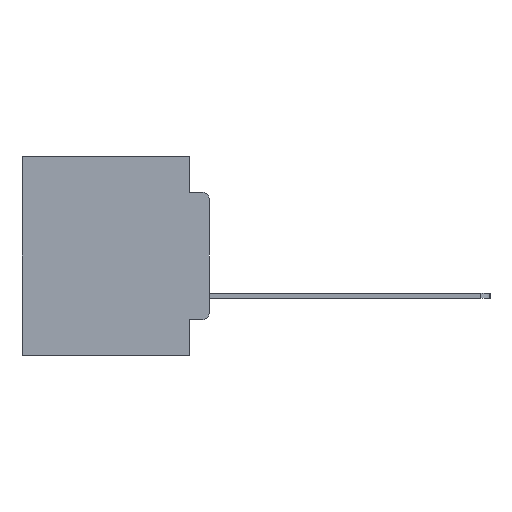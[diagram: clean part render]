
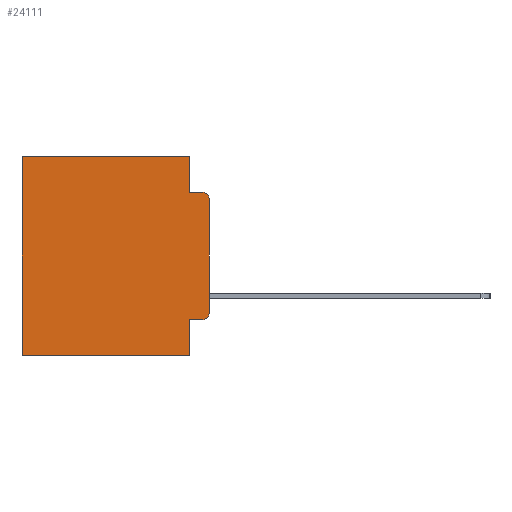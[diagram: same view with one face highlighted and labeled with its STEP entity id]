
A CAD part, left-side view. The second image highlights one B-rep face of the part: STEP entity #24111.
In plain terms, the highlighted planar face has unit normal (-1, 0, 0).
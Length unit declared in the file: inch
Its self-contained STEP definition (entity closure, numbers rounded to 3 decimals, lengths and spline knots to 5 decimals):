
#613 = CIRCLE ( 'NONE', #1823, 0.02 ) ;
#683 = ORIENTED_EDGE ( 'NONE', *, *, #22437, .F. ) ;
#1132 = CARTESIAN_POINT ( 'NONE',  ( 0.298, 0.473, -0.5 ) ) ;
#1179 = LINE ( 'NONE', #14755, #17703 ) ;
#1577 = AXIS2_PLACEMENT_3D ( 'NONE', #6906, #22453, #9178 ) ;
#1823 = AXIS2_PLACEMENT_3D ( 'NONE', #12701, #28021, #14940 ) ;
#1908 = LINE ( 'NONE', #10897, #24934 ) ;
#2142 = ORIENTED_EDGE ( 'NONE', *, *, #2997, .T. ) ;
#2168 = VERTEX_POINT ( 'NONE', #1132 ) ;
#2997 = EDGE_CURVE ( 'NONE', #19765, #2168, #7782, .T. ) ;
#3572 = ORIENTED_EDGE ( 'NONE', *, *, #9066, .F. ) ;
#4216 = DIRECTION ( 'NONE',  ( 0., 1., 0. ) ) ;
#4220 = EDGE_CURVE ( 'NONE', #27204, #19765, #25929, .T. ) ;
#4390 = DIRECTION ( 'NONE',  ( 0., 0., -1. ) ) ;
#4971 = CARTESIAN_POINT ( 'NONE',  ( 0.298, 0., 0. ) ) ;
#5161 = VECTOR ( 'NONE', #7639, 39.37008 ) ;
#5734 = AXIS2_PLACEMENT_3D ( 'NONE', #4971, #20560, #7235 ) ;
#6906 = CARTESIAN_POINT ( 'NONE',  ( 0.298, 0.02, -0.3915 ) ) ;
#7235 = DIRECTION ( 'NONE',  ( 0., 0., -1. ) ) ;
#7298 = CARTESIAN_POINT ( 'NONE',  ( 0.298, 0.051, -0.5 ) ) ;
#7639 = DIRECTION ( 'NONE',  ( 0., 0., -1. ) ) ;
#7782 = LINE ( 'NONE', #15590, #18922 ) ;
#8420 = CARTESIAN_POINT ( 'NONE',  ( 0.298, 0.473, 0. ) ) ;
#8427 = CARTESIAN_POINT ( 'NONE',  ( 0.298, 0.051, -0.0885 ) ) ;
#8883 = EDGE_CURVE ( 'NONE', #19855, #25365, #18760, .T. ) ;
#8916 = VECTOR ( 'NONE', #24172, 39.37008 ) ;
#9066 = EDGE_CURVE ( 'NONE', #27204, #15815, #1908, .T. ) ;
#9178 = DIRECTION ( 'NONE',  ( 0., 0., -1. ) ) ;
#9445 = CARTESIAN_POINT ( 'NONE',  ( 0.298, 0.02, -0.0885 ) ) ;
#9495 = CIRCLE ( 'NONE', #1577, 0.02 ) ;
#10897 = CARTESIAN_POINT ( 'NONE',  ( 0.298, 0.051, 0. ) ) ;
#11019 = ORIENTED_EDGE ( 'NONE', *, *, #20965, .T. ) ;
#11169 = LINE ( 'NONE', #23171, #5161 ) ;
#11352 = ORIENTED_EDGE ( 'NONE', *, *, #26916, .T. ) ;
#12701 = CARTESIAN_POINT ( 'NONE',  ( 0.298, 0.02, -0.1085 ) ) ;
#12762 = ORIENTED_EDGE ( 'NONE', *, *, #19210, .F. ) ;
#14160 = CARTESIAN_POINT ( 'NONE',  ( 0.298, 0., -0.3915 ) ) ;
#14560 = CARTESIAN_POINT ( 'NONE',  ( 0.298, 0.051, 0. ) ) ;
#14755 = CARTESIAN_POINT ( 'NONE',  ( 0.298, 0.051, -0.0885 ) ) ;
#14853 = ORIENTED_EDGE ( 'NONE', *, *, #4220, .T. ) ;
#14940 = DIRECTION ( 'NONE',  ( 0., 0., -1. ) ) ;
#15155 = VECTOR ( 'NONE', #20407, 39.37008 ) ;
#15342 = CARTESIAN_POINT ( 'NONE',  ( 0.298, 0., 0. ) ) ;
#15371 = DIRECTION ( 'NONE',  ( 0., 0., -1. ) ) ;
#15486 = VERTEX_POINT ( 'NONE', #9445 ) ;
#15536 = ORIENTED_EDGE ( 'NONE', *, *, #28252, .F. ) ;
#15590 = CARTESIAN_POINT ( 'NONE',  ( 0.298, 0.473, 0. ) ) ;
#15815 = VERTEX_POINT ( 'NONE', #8427 ) ;
#15839 = LINE ( 'NONE', #18209, #15155 ) ;
#16149 = PLANE ( 'NONE',  #5734 ) ;
#16835 = CARTESIAN_POINT ( 'NONE',  ( 0.298, 0., 0. ) ) ;
#17256 = ORIENTED_EDGE ( 'NONE', *, *, #20653, .T. ) ;
#17289 = CARTESIAN_POINT ( 'NONE',  ( 0.298, 0.02, -0.4115 ) ) ;
#17345 = FACE_OUTER_BOUND ( 'NONE', #27927, .T. ) ;
#17442 = VERTEX_POINT ( 'NONE', #17289 ) ;
#17703 = VECTOR ( 'NONE', #27834, 39.37008 ) ;
#17779 = VERTEX_POINT ( 'NONE', #7298 ) ;
#18069 = VECTOR ( 'NONE', #21240, 39.37008 ) ;
#18209 = CARTESIAN_POINT ( 'NONE',  ( 0.298, 0.051, -0.4115 ) ) ;
#18760 = LINE ( 'NONE', #16835, #18069 ) ;
#18922 = VECTOR ( 'NONE', #4390, 39.37008 ) ;
#19210 = EDGE_CURVE ( 'NONE', #17779, #2168, #27881, .T. ) ;
#19765 = VERTEX_POINT ( 'NONE', #8420 ) ;
#19855 = VERTEX_POINT ( 'NONE', #28456 ) ;
#20407 = DIRECTION ( 'NONE',  ( 0., -1., 0. ) ) ;
#20560 = DIRECTION ( 'NONE',  ( 1., 0., 0. ) ) ;
#20653 = EDGE_CURVE ( 'NONE', #22653, #17442, #15839, .T. ) ;
#20965 = EDGE_CURVE ( 'NONE', #19855, #15486, #613, .T. ) ;
#21240 = DIRECTION ( 'NONE',  ( 0., 0., -1. ) ) ;
#21959 = CARTESIAN_POINT ( 'NONE',  ( 0.298, 0., -0.5 ) ) ;
#22437 = EDGE_CURVE ( 'NONE', #22653, #17779, #11169, .T. ) ;
#22453 = DIRECTION ( 'NONE',  ( -1., 0., 0. ) ) ;
#22653 = VERTEX_POINT ( 'NONE', #23939 ) ;
#22764 = ORIENTED_EDGE ( 'NONE', *, *, #8883, .F. ) ;
#23171 = CARTESIAN_POINT ( 'NONE',  ( 0.298, 0.051, 0. ) ) ;
#23939 = CARTESIAN_POINT ( 'NONE',  ( 0.298, 0.051, -0.4115 ) ) ;
#24111 = ADVANCED_FACE ( 'NONE', ( #17345 ), #16149, .F. ) ;
#24172 = DIRECTION ( 'NONE',  ( 0., 1., 0. ) ) ;
#24934 = VECTOR ( 'NONE', #15371, 39.37008 ) ;
#25250 = VECTOR ( 'NONE', #4216, 39.37008 ) ;
#25365 = VERTEX_POINT ( 'NONE', #14160 ) ;
#25929 = LINE ( 'NONE', #15342, #25250 ) ;
#26916 = EDGE_CURVE ( 'NONE', #17442, #25365, #9495, .T. ) ;
#27204 = VERTEX_POINT ( 'NONE', #14560 ) ;
#27834 = DIRECTION ( 'NONE',  ( 0., -1., 0. ) ) ;
#27881 = LINE ( 'NONE', #21959, #8916 ) ;
#27927 = EDGE_LOOP ( 'NONE', ( #22764, #11019, #15536, #3572, #14853, #2142, #12762, #683, #17256, #11352 ) ) ;
#28021 = DIRECTION ( 'NONE',  ( -1., 0., 0. ) ) ;
#28252 = EDGE_CURVE ( 'NONE', #15815, #15486, #1179, .T. ) ;
#28456 = CARTESIAN_POINT ( 'NONE',  ( 0.298, 0., -0.1085 ) ) ;
